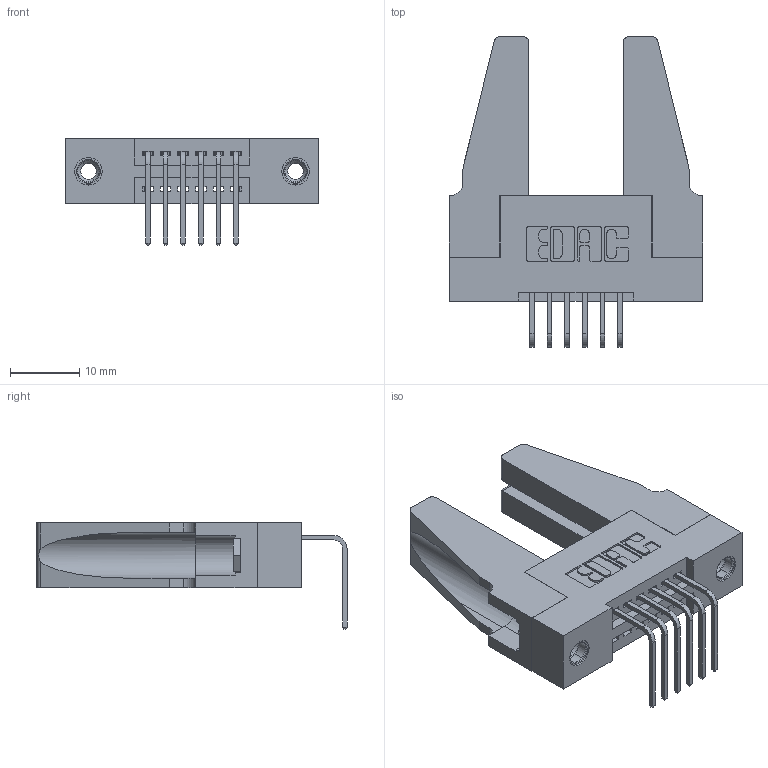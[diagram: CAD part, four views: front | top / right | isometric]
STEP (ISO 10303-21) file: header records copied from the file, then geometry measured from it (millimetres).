
FILE_DESCRIPTION (( 'STEP AP203' ), '1' );
FILE_NAME ('395-006-558-188.STEP', '2019-10-11T01:39:35', ( '' ), ( '' ), 'SwSTEP 2.0', 'SolidWorks 2016', '' );
FILE_SCHEMA (( 'CONFIG_CONTROL_DESIGN' ));
Length unit declared in the file: inch
Products named in the file (5): 345-250-001_345-250-001-102; 345-220-078_345-220-088; 395-006-558-188; 345 Part_Flush Mounting Lugs - 0.156 Dia-TH; 345-292-001_558 Tail - 2
Assembly tree (11 placements, depth 2):
  395-006-558-188
    345 Part_Flush Mounting Lugs - 0.156 Dia-TH
    345-292-001_558 Tail - 2  x6
    345-250-001_345-250-001-102  x2
    345-220-078_345-220-088  x2
Bounding box: 36.47 x 44.69 x 15.37 mm (x, y, z)
Volume: 6442 mm3; surface area: 6996 mm2
Topology: 11 solids, 11 shells, 610 faces, 1747 edges, 1146 vertices
Faces by surface type: plane 404, cylinder 190, cone 12, torus 4
Entity records: 11594 total; most frequent: CARTESIAN_POINT 2000, ORIENTED_EDGE 1900, DIRECTION 1806, EDGE_CURVE 950, VECTOR 752, LINE 752, VERTEX_POINT 626, AXIS2_PLACEMENT_3D 527
